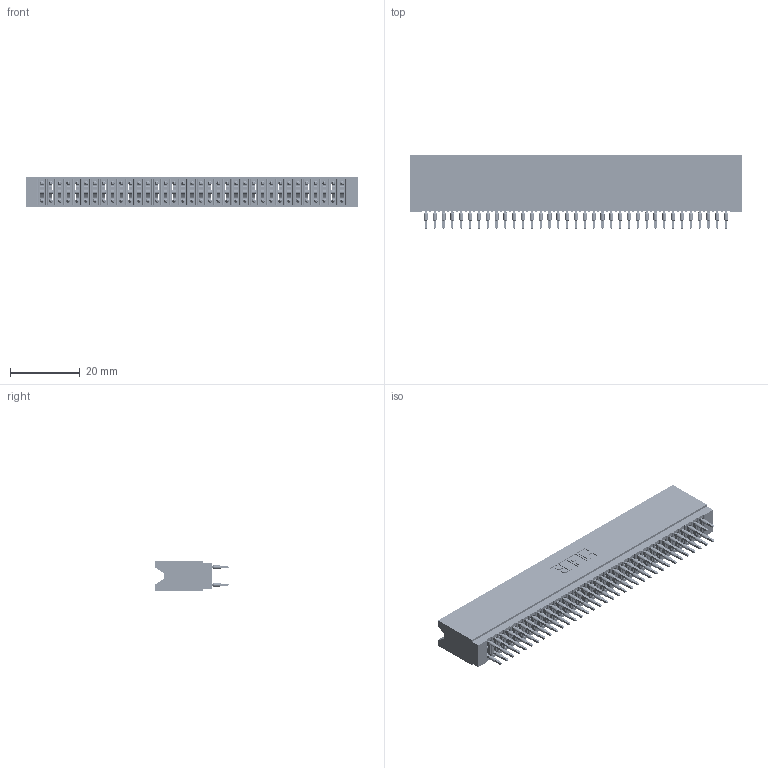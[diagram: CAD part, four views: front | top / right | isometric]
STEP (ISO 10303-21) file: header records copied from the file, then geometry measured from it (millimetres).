
FILE_DESCRIPTION (( 'STEP AP203' ), '1' );
FILE_NAME ('745-070-560-206.STEP', '2026-02-26T19:49:42', ( '' ), ( '' ), 'SwSTEP 2.0', 'SolidWorks 2023', '' );
FILE_SCHEMA (( 'CONFIG_CONTROL_DESIGN' ));
Length unit declared in the file: millimetre
Products named in the file (3): 745-292-001_560; 745-070-560-206; 745 Part_Insulator Option - 06
Assembly tree (71 placements, depth 2):
  745-070-560-206
    745 Part_Insulator Option - 06
    745-292-001_560  x70
Bounding box: 95.5 x 21.22 x 8.89 mm (x, y, z)
Volume: 8879.5 mm3; surface area: 19020.8 mm2
Topology: 71 solids, 71 shells, 6991 faces, 19125 edges, 12142 vertices
Faces by surface type: plane 3626, cylinder 1545, bspline 1400, torus 420
Entity records: 60222 total; most frequent: CARTESIAN_POINT 10952, ORIENTED_EDGE 10374, DIRECTION 9073, EDGE_CURVE 5187, LINE 4787, VECTOR 4787, VERTEX_POINT 3310, AXIS2_PLACEMENT_3D 2143
